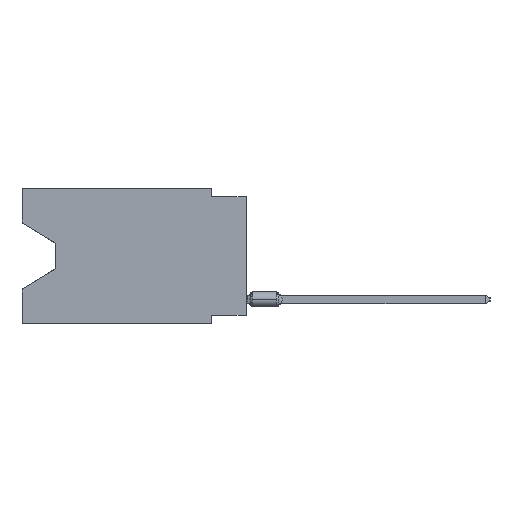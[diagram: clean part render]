
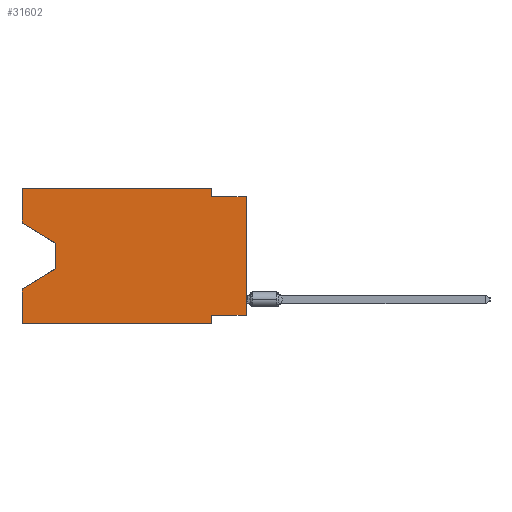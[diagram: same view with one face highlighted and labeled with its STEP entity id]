
A CAD part, left-side view. The second image highlights one B-rep face of the part: STEP entity #31602.
In plain terms, the highlighted planar face has unit normal (-1, 0, 0).
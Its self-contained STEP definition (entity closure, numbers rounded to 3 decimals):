
#120 = LINE ( 'NONE', #806, #31013 ) ;
#706 = CARTESIAN_POINT ( 'NONE',  ( 0., 16.383, -7.36 ) ) ;
#806 = CARTESIAN_POINT ( 'NONE',  ( 0., 16.383, -9.906 ) ) ;
#898 = EDGE_CURVE ( 'NONE', #3733, #18723, #19632, .T. ) ;
#1060 = DIRECTION ( 'NONE',  ( 0., 0., -1. ) ) ;
#2466 = EDGE_CURVE ( 'NONE', #66899, #27541, #36173, .T. ) ;
#3472 = VECTOR ( 'NONE', #16317, 1000. ) ;
#3618 = CARTESIAN_POINT ( 'NONE',  ( 0., 16.383, -9.906 ) ) ;
#3733 = VERTEX_POINT ( 'NONE', #54254 ) ;
#4086 = DIRECTION ( 'NONE',  ( 0., -1., 0. ) ) ;
#4538 = EDGE_CURVE ( 'NONE', #26692, #15793, #43288, .T. ) ;
#5629 = DIRECTION ( 'NONE',  ( 0., -0.855, -0.519 ) ) ;
#5920 = LINE ( 'NONE', #11506, #7387 ) ;
#6673 = EDGE_CURVE ( 'NONE', #54529, #33942, #7211, .T. ) ;
#7211 = LINE ( 'NONE', #59845, #14815 ) ;
#7387 = VECTOR ( 'NONE', #32762, 1000. ) ;
#7454 = CARTESIAN_POINT ( 'NONE',  ( 0., 13.97, -4.013 ) ) ;
#9966 = CARTESIAN_POINT ( 'NONE',  ( 0., 2.54, -0.635 ) ) ;
#10146 = VECTOR ( 'NONE', #56602, 1000. ) ;
#11506 = CARTESIAN_POINT ( 'NONE',  ( 0., 13.97, -4.013 ) ) ;
#12162 = CARTESIAN_POINT ( 'NONE',  ( 0., 2.54, 0. ) ) ;
#12627 = CARTESIAN_POINT ( 'NONE',  ( 0., 0., -9.271 ) ) ;
#14484 = LINE ( 'NONE', #20744, #37214 ) ;
#14815 = VECTOR ( 'NONE', #22882, 1000. ) ;
#15793 = VERTEX_POINT ( 'NONE', #7454 ) ;
#16317 = DIRECTION ( 'NONE',  ( 0., 0., 1. ) ) ;
#16893 = CARTESIAN_POINT ( 'NONE',  ( 0., 2.54, -9.906 ) ) ;
#17349 = CARTESIAN_POINT ( 'NONE',  ( 0., 16.383, 0. ) ) ;
#17432 = PLANE ( 'NONE',  #41133 ) ;
#18357 = ORIENTED_EDGE ( 'NONE', *, *, #31979, .F. ) ;
#18723 = VERTEX_POINT ( 'NONE', #12162 ) ;
#18973 = DIRECTION ( 'NONE',  ( 0., 0., -1. ) ) ;
#19359 = EDGE_CURVE ( 'NONE', #39537, #27541, #53304, .T. ) ;
#19362 = DIRECTION ( 'NONE',  ( 0., 0., 1. ) ) ;
#19632 = LINE ( 'NONE', #66377, #10146 ) ;
#19940 = VECTOR ( 'NONE', #19362, 1000. ) ;
#20377 = VECTOR ( 'NONE', #27012, 1000. ) ;
#20744 = CARTESIAN_POINT ( 'NONE',  ( 0., 0., -9.271 ) ) ;
#22882 = DIRECTION ( 'NONE',  ( 0., 0.855, -0.519 ) ) ;
#23951 = CARTESIAN_POINT ( 'NONE',  ( 0., 0., -0.635 ) ) ;
#24378 = VECTOR ( 'NONE', #18973, 1000. ) ;
#25259 = LINE ( 'NONE', #46552, #19940 ) ;
#25730 = ORIENTED_EDGE ( 'NONE', *, *, #38656, .F. ) ;
#26692 = VERTEX_POINT ( 'NONE', #56222 ) ;
#27012 = DIRECTION ( 'NONE',  ( 0., 0., -1. ) ) ;
#27195 = ORIENTED_EDGE ( 'NONE', *, *, #4538, .T. ) ;
#27541 = VERTEX_POINT ( 'NONE', #23951 ) ;
#30215 = EDGE_CURVE ( 'NONE', #41905, #48305, #120, .T. ) ;
#31013 = VECTOR ( 'NONE', #36756, 1000. ) ;
#31602 = ADVANCED_FACE ( 'NONE', ( #33130 ), #17432, .F. ) ;
#31979 = EDGE_CURVE ( 'NONE', #26692, #3733, #54672, .T. ) ;
#32444 = DIRECTION ( 'NONE',  ( 1., 0., 0. ) ) ;
#32718 = VERTEX_POINT ( 'NONE', #37923 ) ;
#32762 = DIRECTION ( 'NONE',  ( 0., 0., -1. ) ) ;
#33130 = FACE_OUTER_BOUND ( 'NONE', #36535, .T. ) ;
#33351 = ORIENTED_EDGE ( 'NONE', *, *, #46192, .F. ) ;
#33942 = VERTEX_POINT ( 'NONE', #706 ) ;
#36173 = LINE ( 'NONE', #45942, #41482 ) ;
#36535 = EDGE_LOOP ( 'NONE', ( #27195, #52480, #67453, #33351, #37556, #63701, #43703, #68662, #61854, #25730, #64279, #18357 ) ) ;
#36756 = DIRECTION ( 'NONE',  ( 0., -1., 0. ) ) ;
#37214 = VECTOR ( 'NONE', #57027, 1000. ) ;
#37556 = ORIENTED_EDGE ( 'NONE', *, *, #30215, .T. ) ;
#37683 = CARTESIAN_POINT ( 'NONE',  ( 0., 16.383, 0. ) ) ;
#37923 = CARTESIAN_POINT ( 'NONE',  ( 0., 2.54, -9.271 ) ) ;
#38656 = EDGE_CURVE ( 'NONE', #18723, #66899, #45463, .T. ) ;
#39537 = VERTEX_POINT ( 'NONE', #12627 ) ;
#41133 = AXIS2_PLACEMENT_3D ( 'NONE', #37683, #32444, #1060 ) ;
#41482 = VECTOR ( 'NONE', #4086, 1000. ) ;
#41905 = VERTEX_POINT ( 'NONE', #3618 ) ;
#42031 = LINE ( 'NONE', #16893, #20377 ) ;
#43213 = CARTESIAN_POINT ( 'NONE',  ( 0., 13.97, -5.893 ) ) ;
#43288 = LINE ( 'NONE', #53409, #60942 ) ;
#43703 = ORIENTED_EDGE ( 'NONE', *, *, #45378, .F. ) ;
#45378 = EDGE_CURVE ( 'NONE', #39537, #32718, #14484, .T. ) ;
#45463 = LINE ( 'NONE', #66737, #24378 ) ;
#45942 = CARTESIAN_POINT ( 'NONE',  ( 0., 0., -0.635 ) ) ;
#46192 = EDGE_CURVE ( 'NONE', #41905, #33942, #25259, .T. ) ;
#46552 = CARTESIAN_POINT ( 'NONE',  ( 0., 16.383, 0. ) ) ;
#48305 = VERTEX_POINT ( 'NONE', #62229 ) ;
#52221 = EDGE_CURVE ( 'NONE', #32718, #48305, #42031, .T. ) ;
#52480 = ORIENTED_EDGE ( 'NONE', *, *, #55627, .T. ) ;
#53304 = LINE ( 'NONE', #53652, #57026 ) ;
#53409 = CARTESIAN_POINT ( 'NONE',  ( 0., 16.383, -2.546 ) ) ;
#53652 = CARTESIAN_POINT ( 'NONE',  ( 0., 0., 0. ) ) ;
#54254 = CARTESIAN_POINT ( 'NONE',  ( 0., 16.383, 0. ) ) ;
#54529 = VERTEX_POINT ( 'NONE', #43213 ) ;
#54672 = LINE ( 'NONE', #17349, #3472 ) ;
#55627 = EDGE_CURVE ( 'NONE', #15793, #54529, #5920, .T. ) ;
#56222 = CARTESIAN_POINT ( 'NONE',  ( 0., 16.383, -2.546 ) ) ;
#56602 = DIRECTION ( 'NONE',  ( 0., -1., 0. ) ) ;
#57026 = VECTOR ( 'NONE', #64112, 1000. ) ;
#57027 = DIRECTION ( 'NONE',  ( 0., 1., 0. ) ) ;
#59845 = CARTESIAN_POINT ( 'NONE',  ( 0., 13.97, -5.893 ) ) ;
#60942 = VECTOR ( 'NONE', #5629, 1000. ) ;
#61854 = ORIENTED_EDGE ( 'NONE', *, *, #2466, .F. ) ;
#62229 = CARTESIAN_POINT ( 'NONE',  ( 0., 2.54, -9.906 ) ) ;
#63701 = ORIENTED_EDGE ( 'NONE', *, *, #52221, .F. ) ;
#64112 = DIRECTION ( 'NONE',  ( 0., 0., 1. ) ) ;
#64279 = ORIENTED_EDGE ( 'NONE', *, *, #898, .F. ) ;
#66377 = CARTESIAN_POINT ( 'NONE',  ( 0., 16.383, 0. ) ) ;
#66737 = CARTESIAN_POINT ( 'NONE',  ( 0., 2.54, 0. ) ) ;
#66899 = VERTEX_POINT ( 'NONE', #9966 ) ;
#67453 = ORIENTED_EDGE ( 'NONE', *, *, #6673, .T. ) ;
#68662 = ORIENTED_EDGE ( 'NONE', *, *, #19359, .T. ) ;
